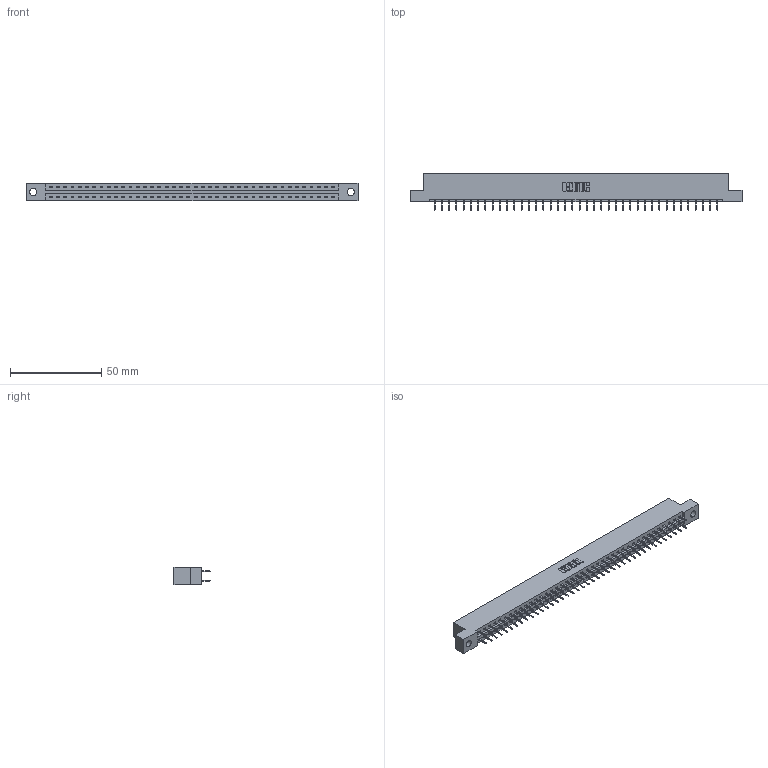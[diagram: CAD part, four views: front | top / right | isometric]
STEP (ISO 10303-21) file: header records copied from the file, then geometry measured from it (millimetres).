
FILE_DESCRIPTION (( 'STEP AP203' ), '1' );
FILE_NAME ('337-080-524-204.STEP', '2018-08-12T17:47:30', ( '' ), ( '' ), 'SwSTEP 2.0', 'SolidWorks 2016', '' );
FILE_SCHEMA (( 'CONFIG_CONTROL_DESIGN' ));
Length unit declared in the file: inch
Products named in the file (3): 337 Part_Flush Mounting Lugs - 0.156 Dia-TH; 345-292-001_345-293-124; 337-080-524-204
Assembly tree (81 placements, depth 2):
  337-080-524-204
    337 Part_Flush Mounting Lugs - 0.156 Dia-TH
    345-292-001_345-293-124  x80
Bounding box: 181.51 x 19.69 x 9.4 mm (x, y, z)
Volume: 18893.3 mm3; surface area: 20761.9 mm2
Topology: 81 solids, 81 shells, 4754 faces, 13511 edges, 8686 vertices
Faces by surface type: plane 3590, cylinder 1164
Entity records: 31349 total; most frequent: CARTESIAN_POINT 5282, ORIENTED_EDGE 5218, DIRECTION 4497, EDGE_CURVE 2609, LINE 2485, VECTOR 2485, VERTEX_POINT 1734, AXIS2_PLACEMENT_3D 1006
